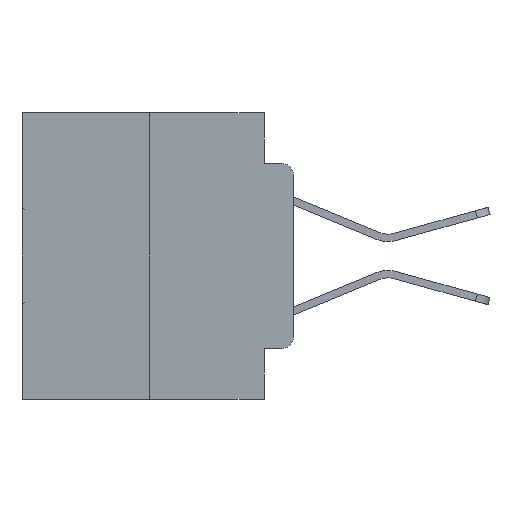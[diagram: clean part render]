
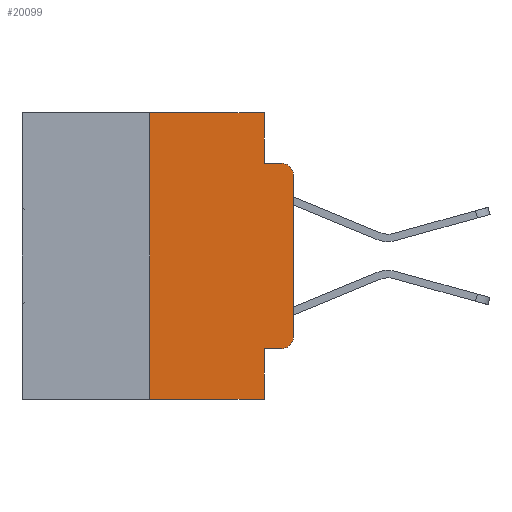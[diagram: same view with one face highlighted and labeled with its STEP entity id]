
A CAD part, left-side view. The second image highlights one B-rep face of the part: STEP entity #20099.
In plain terms, the highlighted planar face has unit normal (-1, 0, 0).
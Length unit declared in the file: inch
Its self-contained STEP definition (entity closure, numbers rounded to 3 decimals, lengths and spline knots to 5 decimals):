
#35 = DIRECTION ( 'NONE',  ( 0., -1., 0. ) ) ;
#90 = VERTEX_POINT ( 'NONE', #4732 ) ;
#92 = EDGE_CURVE ( 'NONE', #16575, #9592, #21318, .T. ) ;
#493 = VECTOR ( 'NONE', #35, 39.37008 ) ;
#568 = CARTESIAN_POINT ( 'NONE',  ( 0., 0.473, 0. ) ) ;
#1667 = DIRECTION ( 'NONE',  ( 0., -1., 0. ) ) ;
#2139 = EDGE_CURVE ( 'NONE', #9592, #8283, #13938, .T. ) ;
#2228 = DIRECTION ( 'NONE',  ( -1., 0., 0. ) ) ;
#2507 = DIRECTION ( 'NONE',  ( 0., 0., 1. ) ) ;
#2863 = FACE_OUTER_BOUND ( 'NONE', #26555, .T. ) ;
#2953 = AXIS2_PLACEMENT_3D ( 'NONE', #28520, #2228, #23879 ) ;
#2997 = EDGE_CURVE ( 'NONE', #11982, #25438, #7875, .T. ) ;
#3537 = EDGE_CURVE ( 'NONE', #6429, #90, #28680, .T. ) ;
#3734 = ORIENTED_EDGE ( 'NONE', *, *, #16403, .F. ) ;
#3825 = LINE ( 'NONE', #13229, #21976 ) ;
#4274 = CARTESIAN_POINT ( 'NONE',  ( 0., 0.051, -0.0885 ) ) ;
#4318 = VECTOR ( 'NONE', #9297, 39.37008 ) ;
#4376 = CARTESIAN_POINT ( 'NONE',  ( 0., 0.051, 0. ) ) ;
#4652 = CARTESIAN_POINT ( 'NONE',  ( 0., 0.051, -0.4115 ) ) ;
#4732 = CARTESIAN_POINT ( 'NONE',  ( 0., 0.051, -0.5 ) ) ;
#5121 = LINE ( 'NONE', #14539, #493 ) ;
#5384 = VERTEX_POINT ( 'NONE', #11317 ) ;
#6021 = EDGE_CURVE ( 'NONE', #6429, #11982, #26162, .T. ) ;
#6429 = VERTEX_POINT ( 'NONE', #18385 ) ;
#6857 = EDGE_CURVE ( 'NONE', #25527, #5384, #11313, .T. ) ;
#7709 = CARTESIAN_POINT ( 'NONE',  ( 0., 0.02, -0.4115 ) ) ;
#7875 = CIRCLE ( 'NONE', #15266, 0.02 ) ;
#8283 = VERTEX_POINT ( 'NONE', #4274 ) ;
#9297 = DIRECTION ( 'NONE',  ( 0., 0., -1. ) ) ;
#9500 = CARTESIAN_POINT ( 'NONE',  ( 0., 0.02, -0.3915 ) ) ;
#9592 = VERTEX_POINT ( 'NONE', #25905 ) ;
#9987 = EDGE_CURVE ( 'NONE', #13919, #90, #5121, .T. ) ;
#10684 = ORIENTED_EDGE ( 'NONE', *, *, #2997, .T. ) ;
#11257 = DIRECTION ( 'NONE',  ( 0., 0., 1. ) ) ;
#11313 = CIRCLE ( 'NONE', #2953, 0.02 ) ;
#11317 = CARTESIAN_POINT ( 'NONE',  ( 0., 0.02, -0.0885 ) ) ;
#11557 = EDGE_CURVE ( 'NONE', #25438, #25527, #13115, .T. ) ;
#11732 = DIRECTION ( 'NONE',  ( 0., -1., 0. ) ) ;
#11982 = VERTEX_POINT ( 'NONE', #7709 ) ;
#12052 = VECTOR ( 'NONE', #28415, 39.37008 ) ;
#12566 = DIRECTION ( 'NONE',  ( 0., 0., -1. ) ) ;
#13115 = LINE ( 'NONE', #30031, #17841 ) ;
#13188 = ORIENTED_EDGE ( 'NONE', *, *, #2139, .F. ) ;
#13229 = CARTESIAN_POINT ( 'NONE',  ( 0., 0.051, -0.0885 ) ) ;
#13919 = VERTEX_POINT ( 'NONE', #21821 ) ;
#13938 = LINE ( 'NONE', #4376, #4318 ) ;
#13990 = CARTESIAN_POINT ( 'NONE',  ( 0., 0.473, 0. ) ) ;
#14153 = ORIENTED_EDGE ( 'NONE', *, *, #3537, .F. ) ;
#14539 = CARTESIAN_POINT ( 'NONE',  ( 0., 0.473, -0.5 ) ) ;
#14921 = ORIENTED_EDGE ( 'NONE', *, *, #6857, .T. ) ;
#14975 = CARTESIAN_POINT ( 'NONE',  ( 0., 0., -0.3915 ) ) ;
#15266 = AXIS2_PLACEMENT_3D ( 'NONE', #9500, #21463, #23768 ) ;
#16403 = EDGE_CURVE ( 'NONE', #13919, #16575, #21247, .T. ) ;
#16575 = VERTEX_POINT ( 'NONE', #29120 ) ;
#16899 = DIRECTION ( 'NONE',  ( 0., 0., -1. ) ) ;
#17538 = PLANE ( 'NONE',  #28590 ) ;
#17841 = VECTOR ( 'NONE', #11257, 39.37008 ) ;
#18385 = CARTESIAN_POINT ( 'NONE',  ( 0., 0.051, -0.4115 ) ) ;
#20099 = ADVANCED_FACE ( 'NONE', ( #2863 ), #17538, .F. ) ;
#20520 = ORIENTED_EDGE ( 'NONE', *, *, #27037, .F. ) ;
#20827 = ORIENTED_EDGE ( 'NONE', *, *, #92, .F. ) ;
#21247 = LINE ( 'NONE', #28496, #25154 ) ;
#21318 = LINE ( 'NONE', #13990, #12052 ) ;
#21463 = DIRECTION ( 'NONE',  ( -1., 0., 0. ) ) ;
#21821 = CARTESIAN_POINT ( 'NONE',  ( 0., 0.25, -0.5 ) ) ;
#21976 = VECTOR ( 'NONE', #1667, 39.37008 ) ;
#23768 = DIRECTION ( 'NONE',  ( 0., 0., -1. ) ) ;
#23879 = DIRECTION ( 'NONE',  ( 0., 0., -1. ) ) ;
#24288 = CARTESIAN_POINT ( 'NONE',  ( 0., 0., -0.1085 ) ) ;
#24521 = DIRECTION ( 'NONE',  ( 1., 0., 0. ) ) ;
#24571 = ORIENTED_EDGE ( 'NONE', *, *, #6021, .T. ) ;
#25154 = VECTOR ( 'NONE', #2507, 39.37008 ) ;
#25438 = VERTEX_POINT ( 'NONE', #14975 ) ;
#25527 = VERTEX_POINT ( 'NONE', #24288 ) ;
#25890 = VECTOR ( 'NONE', #11732, 39.37008 ) ;
#25905 = CARTESIAN_POINT ( 'NONE',  ( 0., 0.051, 0. ) ) ;
#26162 = LINE ( 'NONE', #4652, #25890 ) ;
#26203 = CARTESIAN_POINT ( 'NONE',  ( 0., 0.051, 0. ) ) ;
#26555 = EDGE_LOOP ( 'NONE', ( #30122, #14921, #20520, #13188, #20827, #3734, #27763, #14153, #24571, #10684 ) ) ;
#27037 = EDGE_CURVE ( 'NONE', #8283, #5384, #3825, .T. ) ;
#27763 = ORIENTED_EDGE ( 'NONE', *, *, #9987, .T. ) ;
#28415 = DIRECTION ( 'NONE',  ( 0., -1., 0. ) ) ;
#28496 = CARTESIAN_POINT ( 'NONE',  ( 0., 0.25, 0. ) ) ;
#28520 = CARTESIAN_POINT ( 'NONE',  ( 0., 0.02, -0.1085 ) ) ;
#28590 = AXIS2_PLACEMENT_3D ( 'NONE', #568, #24521, #12566 ) ;
#28609 = VECTOR ( 'NONE', #16899, 39.37008 ) ;
#28680 = LINE ( 'NONE', #26203, #28609 ) ;
#29120 = CARTESIAN_POINT ( 'NONE',  ( 0., 0.25, 0. ) ) ;
#30031 = CARTESIAN_POINT ( 'NONE',  ( 0., 0., 0. ) ) ;
#30122 = ORIENTED_EDGE ( 'NONE', *, *, #11557, .T. ) ;
